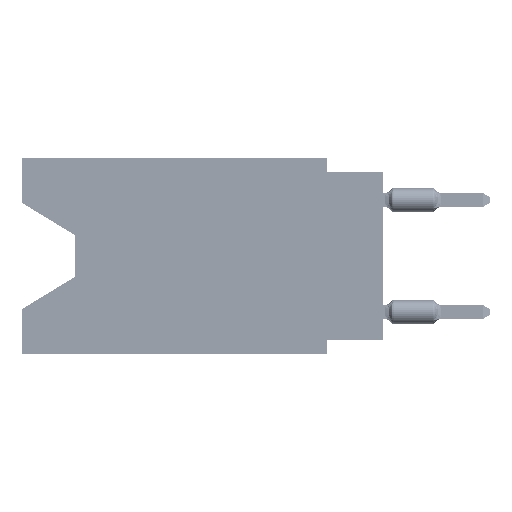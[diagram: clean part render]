
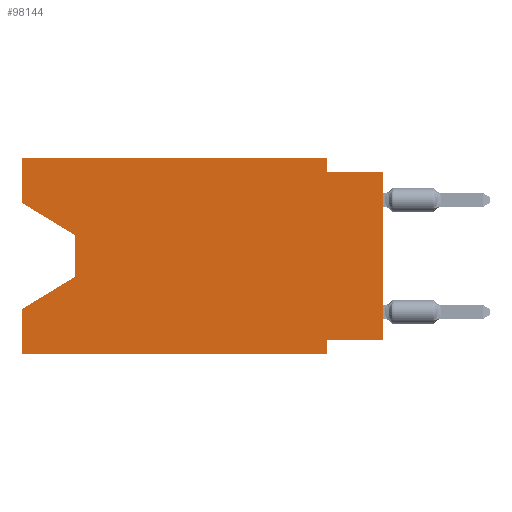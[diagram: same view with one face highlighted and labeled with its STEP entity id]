
A CAD part, left-side view. The second image highlights one B-rep face of the part: STEP entity #98144.
In plain terms, the highlighted planar face has unit normal (-1, 0, 0).
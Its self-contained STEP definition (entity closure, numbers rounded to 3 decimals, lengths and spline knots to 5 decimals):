
#242 = CARTESIAN_POINT ( 'NONE',  ( 0., 0., -0.325 ) ) ;
#486 = DIRECTION ( 'NONE',  ( 0., -1., 0. ) ) ;
#894 = EDGE_CURVE ( 'NONE', #29535, #8150, #97233, .T. ) ;
#2376 = VERTEX_POINT ( 'NONE', #56625 ) ;
#2616 = ORIENTED_EDGE ( 'NONE', *, *, #61871, .T. ) ;
#3538 = VECTOR ( 'NONE', #42930, 39.37008 ) ;
#4067 = EDGE_CURVE ( 'NONE', #77259, #81608, #55612, .T. ) ;
#5184 = CARTESIAN_POINT ( 'NONE',  ( 0., 0., 0. ) ) ;
#6390 = LINE ( 'NONE', #57431, #3538 ) ;
#8150 = VERTEX_POINT ( 'NONE', #36369 ) ;
#8611 = ORIENTED_EDGE ( 'NONE', *, *, #48078, .F. ) ;
#9914 = EDGE_CURVE ( 'NONE', #71608, #75231, #82776, .T. ) ;
#11006 = ORIENTED_EDGE ( 'NONE', *, *, #4067, .F. ) ;
#11717 = VECTOR ( 'NONE', #74769, 39.37008 ) ;
#13470 = FACE_OUTER_BOUND ( 'NONE', #97853, .T. ) ;
#15363 = CARTESIAN_POINT ( 'NONE',  ( 0., 0.645, 0. ) ) ;
#15765 = VECTOR ( 'NONE', #65214, 39.37008 ) ;
#16016 = CARTESIAN_POINT ( 'NONE',  ( 0., 0.1, -0.325 ) ) ;
#16535 = VECTOR ( 'NONE', #36876, 39.37008 ) ;
#18095 = CARTESIAN_POINT ( 'NONE',  ( 0., 0.1, -0.35 ) ) ;
#20561 = VERTEX_POINT ( 'NONE', #74890 ) ;
#20665 = LINE ( 'NONE', #79719, #43386 ) ;
#22055 = VERTEX_POINT ( 'NONE', #61389 ) ;
#22401 = VERTEX_POINT ( 'NONE', #96338 ) ;
#22729 = CARTESIAN_POINT ( 'NONE',  ( 0., 0.55, -0.212 ) ) ;
#25085 = VECTOR ( 'NONE', #42596, 39.37008 ) ;
#25587 = CARTESIAN_POINT ( 'NONE',  ( 0., 0.1, -0.35 ) ) ;
#27971 = EDGE_CURVE ( 'NONE', #22055, #37812, #84777, .T. ) ;
#28600 = EDGE_CURVE ( 'NONE', #20561, #81608, #45023, .T. ) ;
#29535 = VERTEX_POINT ( 'NONE', #242 ) ;
#29939 = PLANE ( 'NONE',  #66526 ) ;
#31090 = VECTOR ( 'NONE', #78074, 39.37008 ) ;
#36369 = CARTESIAN_POINT ( 'NONE',  ( 0., 0., -0.025 ) ) ;
#36876 = DIRECTION ( 'NONE',  ( 0., 0., 1. ) ) ;
#37812 = VERTEX_POINT ( 'NONE', #38904 ) ;
#37864 = LINE ( 'NONE', #98893, #16535 ) ;
#38904 = CARTESIAN_POINT ( 'NONE',  ( 0., 0.1, -0.025 ) ) ;
#39245 = CARTESIAN_POINT ( 'NONE',  ( 0., 0.1, 0. ) ) ;
#41863 = CARTESIAN_POINT ( 'NONE',  ( 0., 0.55, -0.212 ) ) ;
#41911 = ORIENTED_EDGE ( 'NONE', *, *, #28600, .T. ) ;
#42596 = DIRECTION ( 'NONE',  ( 0., -0.855, -0.519 ) ) ;
#42930 = DIRECTION ( 'NONE',  ( 0., 0., 1. ) ) ;
#43386 = VECTOR ( 'NONE', #50170, 39.37008 ) ;
#43922 = ORIENTED_EDGE ( 'NONE', *, *, #65926, .T. ) ;
#45023 = LINE ( 'NONE', #61024, #78297 ) ;
#45437 = EDGE_CURVE ( 'NONE', #20561, #75231, #37864, .T. ) ;
#48038 = DIRECTION ( 'NONE',  ( 0., 0., -1. ) ) ;
#48078 = EDGE_CURVE ( 'NONE', #37812, #8150, #49029, .T. ) ;
#49029 = LINE ( 'NONE', #72046, #31090 ) ;
#50170 = DIRECTION ( 'NONE',  ( 0., 1., 0. ) ) ;
#51980 = DIRECTION ( 'NONE',  ( 0., 0., -1. ) ) ;
#53064 = ORIENTED_EDGE ( 'NONE', *, *, #53106, .F. ) ;
#53106 = EDGE_CURVE ( 'NONE', #29535, #77259, #20665, .T. ) ;
#53602 = EDGE_CURVE ( 'NONE', #79419, #22401, #6390, .T. ) ;
#55612 = LINE ( 'NONE', #18095, #86899 ) ;
#56002 = ORIENTED_EDGE ( 'NONE', *, *, #894, .T. ) ;
#56625 = CARTESIAN_POINT ( 'NONE',  ( 0., 0.55, -0.138 ) ) ;
#57431 = CARTESIAN_POINT ( 'NONE',  ( 0., 0.645, 0. ) ) ;
#58257 = EDGE_CURVE ( 'NONE', #22401, #22055, #69363, .T. ) ;
#61024 = CARTESIAN_POINT ( 'NONE',  ( 0., 0.645, -0.35 ) ) ;
#61389 = CARTESIAN_POINT ( 'NONE',  ( 0., 0.1, 0. ) ) ;
#61871 = EDGE_CURVE ( 'NONE', #79419, #2376, #89626, .T. ) ;
#65214 = DIRECTION ( 'NONE',  ( 0., 0., 1. ) ) ;
#65926 = EDGE_CURVE ( 'NONE', #2376, #71608, #76601, .T. ) ;
#66526 = AXIS2_PLACEMENT_3D ( 'NONE', #82005, #91987, #51980 ) ;
#69363 = LINE ( 'NONE', #15363, #96595 ) ;
#71225 = ORIENTED_EDGE ( 'NONE', *, *, #27971, .F. ) ;
#71229 = CARTESIAN_POINT ( 'NONE',  ( 0., 0.645, -0.26975 ) ) ;
#71608 = VERTEX_POINT ( 'NONE', #41863 ) ;
#72046 = CARTESIAN_POINT ( 'NONE',  ( 0., 0., -0.025 ) ) ;
#74293 = ORIENTED_EDGE ( 'NONE', *, *, #58257, .F. ) ;
#74769 = DIRECTION ( 'NONE',  ( 0., 0.855, -0.519 ) ) ;
#74890 = CARTESIAN_POINT ( 'NONE',  ( 0., 0.645, -0.35 ) ) ;
#75231 = VERTEX_POINT ( 'NONE', #71229 ) ;
#76601 = LINE ( 'NONE', #85101, #86219 ) ;
#77259 = VERTEX_POINT ( 'NONE', #16016 ) ;
#77268 = DIRECTION ( 'NONE',  ( 0., 0., -1. ) ) ;
#78074 = DIRECTION ( 'NONE',  ( 0., -1., 0. ) ) ;
#78297 = VECTOR ( 'NONE', #486, 39.37008 ) ;
#78829 = CARTESIAN_POINT ( 'NONE',  ( 0., 0.645, -0.08025 ) ) ;
#79419 = VERTEX_POINT ( 'NONE', #78829 ) ;
#79719 = CARTESIAN_POINT ( 'NONE',  ( 0., 0., -0.325 ) ) ;
#81608 = VERTEX_POINT ( 'NONE', #25587 ) ;
#81621 = CARTESIAN_POINT ( 'NONE',  ( 0., 0.645, -0.08025 ) ) ;
#82005 = CARTESIAN_POINT ( 'NONE',  ( 0., 0.645, 0. ) ) ;
#82213 = ORIENTED_EDGE ( 'NONE', *, *, #53602, .F. ) ;
#82776 = LINE ( 'NONE', #22729, #11717 ) ;
#83015 = VECTOR ( 'NONE', #77268, 39.37008 ) ;
#84777 = LINE ( 'NONE', #39245, #83015 ) ;
#85101 = CARTESIAN_POINT ( 'NONE',  ( 0., 0.55, -0.138 ) ) ;
#86219 = VECTOR ( 'NONE', #48038, 39.37008 ) ;
#86248 = ORIENTED_EDGE ( 'NONE', *, *, #9914, .T. ) ;
#86899 = VECTOR ( 'NONE', #95148, 39.37008 ) ;
#89626 = LINE ( 'NONE', #81621, #25085 ) ;
#90922 = DIRECTION ( 'NONE',  ( 0., -1., 0. ) ) ;
#91987 = DIRECTION ( 'NONE',  ( 1., 0., 0. ) ) ;
#94314 = ORIENTED_EDGE ( 'NONE', *, *, #45437, .F. ) ;
#95148 = DIRECTION ( 'NONE',  ( 0., 0., -1. ) ) ;
#96338 = CARTESIAN_POINT ( 'NONE',  ( 0., 0.645, 0. ) ) ;
#96595 = VECTOR ( 'NONE', #90922, 39.37008 ) ;
#97233 = LINE ( 'NONE', #5184, #15765 ) ;
#97853 = EDGE_LOOP ( 'NONE', ( #2616, #43922, #86248, #94314, #41911, #11006, #53064, #56002, #8611, #71225, #74293, #82213 ) ) ;
#98144 = ADVANCED_FACE ( 'NONE', ( #13470 ), #29939, .F. ) ;
#98893 = CARTESIAN_POINT ( 'NONE',  ( 0., 0.645, 0. ) ) ;
